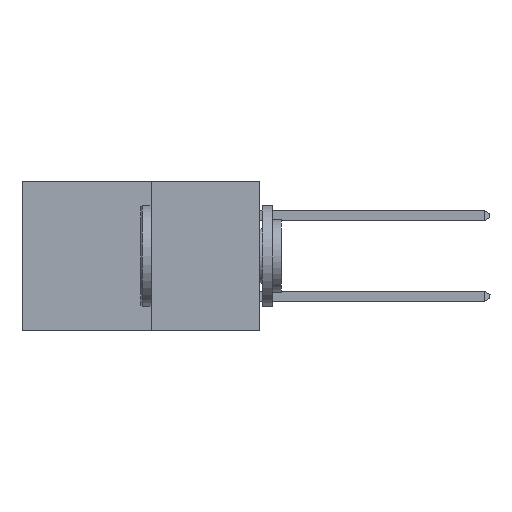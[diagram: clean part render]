
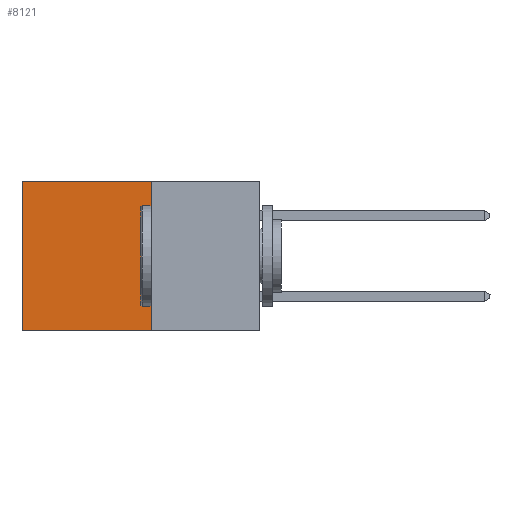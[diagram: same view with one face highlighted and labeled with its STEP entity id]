
A CAD part, left-side view. The second image highlights one B-rep face of the part: STEP entity #8121.
In plain terms, the highlighted planar face has unit normal (-1, 0, 0).
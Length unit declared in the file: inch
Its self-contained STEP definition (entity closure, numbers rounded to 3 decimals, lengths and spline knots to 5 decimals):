
#350 = DIRECTION ( 'NONE',  ( 0., 0., -1. ) ) ;
#1020 = AXIS2_PLACEMENT_3D ( 'NONE', #10063, #5280, #350 ) ;
#1049 = LINE ( 'NONE', #7504, #5149 ) ;
#1285 = EDGE_CURVE ( 'NONE', #2793, #2644, #4805, .T. ) ;
#1470 = EDGE_CURVE ( 'NONE', #5750, #3805, #8546, .T. ) ;
#1536 = DIRECTION ( 'NONE',  ( 0., 1., 0. ) ) ;
#1826 = CARTESIAN_POINT ( 'NONE',  ( 0.277, 0.59, 0. ) ) ;
#1856 = VECTOR ( 'NONE', #8837, 39.37008 ) ;
#2026 = CARTESIAN_POINT ( 'NONE',  ( 0.277, 0.59, -0.37 ) ) ;
#2609 = VECTOR ( 'NONE', #9709, 39.37008 ) ;
#2644 = VERTEX_POINT ( 'NONE', #2026 ) ;
#2793 = VERTEX_POINT ( 'NONE', #3628 ) ;
#3192 = ORIENTED_EDGE ( 'NONE', *, *, #1470, .T. ) ;
#3628 = CARTESIAN_POINT ( 'NONE',  ( 0.277, 0.27, -0.37 ) ) ;
#3680 = PLANE ( 'NONE',  #1020 ) ;
#3781 = EDGE_CURVE ( 'NONE', #3805, #2644, #4056, .T. ) ;
#3805 = VERTEX_POINT ( 'NONE', #1826 ) ;
#4056 = LINE ( 'NONE', #9826, #1856 ) ;
#4502 = ORIENTED_EDGE ( 'NONE', *, *, #3781, .T. ) ;
#4747 = VECTOR ( 'NONE', #1536, 39.37008 ) ;
#4805 = LINE ( 'NONE', #10261, #2609 ) ;
#4926 = FACE_OUTER_BOUND ( 'NONE', #10473, .T. ) ;
#5149 = VECTOR ( 'NONE', #7461, 39.37008 ) ;
#5280 = DIRECTION ( 'NONE',  ( 1., 0., 0. ) ) ;
#5750 = VERTEX_POINT ( 'NONE', #9002 ) ;
#5925 = EDGE_CURVE ( 'NONE', #5750, #2793, #1049, .T. ) ;
#7461 = DIRECTION ( 'NONE',  ( 0., 0., -1. ) ) ;
#7504 = CARTESIAN_POINT ( 'NONE',  ( 0.277, 0.27, -0.37 ) ) ;
#8116 = CARTESIAN_POINT ( 'NONE',  ( 0.277, 0.27, 0. ) ) ;
#8121 = ADVANCED_FACE ( 'NONE', ( #4926 ), #3680, .F. ) ;
#8546 = LINE ( 'NONE', #8116, #4747 ) ;
#8837 = DIRECTION ( 'NONE',  ( 0., 0., -1. ) ) ;
#9002 = CARTESIAN_POINT ( 'NONE',  ( 0.277, 0.27, 0. ) ) ;
#9214 = ORIENTED_EDGE ( 'NONE', *, *, #1285, .F. ) ;
#9709 = DIRECTION ( 'NONE',  ( 0., 1., 0. ) ) ;
#9826 = CARTESIAN_POINT ( 'NONE',  ( 0.277, 0.59, -0.37 ) ) ;
#10054 = ORIENTED_EDGE ( 'NONE', *, *, #5925, .F. ) ;
#10063 = CARTESIAN_POINT ( 'NONE',  ( 0.277, 0.27, -0.37 ) ) ;
#10261 = CARTESIAN_POINT ( 'NONE',  ( 0.277, 0.27, -0.37 ) ) ;
#10473 = EDGE_LOOP ( 'NONE', ( #4502, #9214, #10054, #3192 ) ) ;
